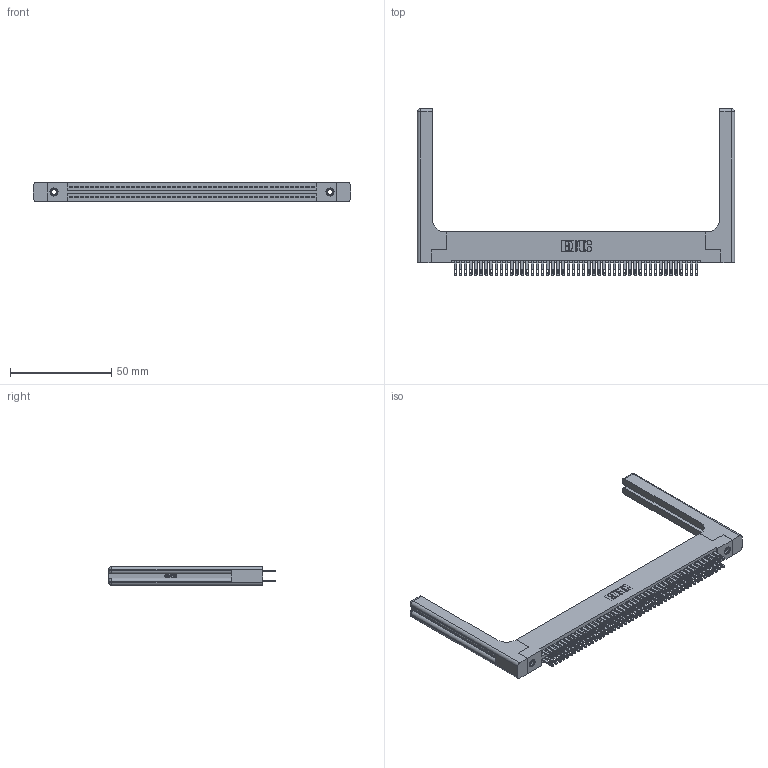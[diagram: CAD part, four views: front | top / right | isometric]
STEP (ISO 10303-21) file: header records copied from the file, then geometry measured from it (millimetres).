
FILE_DESCRIPTION (( 'STEP AP203' ), '1' );
FILE_NAME ('345-096-500-258.STEP', '2019-11-02T06:30:21', ( '' ), ( '' ), 'SwSTEP 2.0', 'SolidWorks 2016', '' );
FILE_SCHEMA (( 'CONFIG_CONTROL_DESIGN' ));
Length unit declared in the file: inch
Products named in the file (5): 345-096-500-258; 345 Part_Flush Mounting Lugs - 0.156 Dia-TH; 345-292-001_345-293-100; 345-220-058_345-220-058; 345-250-001_345-250-001-102
Assembly tree (101 placements, depth 2):
  345-096-500-258
    345 Part_Flush Mounting Lugs - 0.156 Dia-TH
    345-292-001_345-293-100  x96
    345-250-001_345-250-001-102  x2
    345-220-058_345-220-058  x2
Bounding box: 156.95 x 82.47 x 9.4 mm (x, y, z)
Volume: 24070.1 mm3; surface area: 29206.3 mm2
Topology: 101 solids, 101 shells, 4798 faces, 14543 edges, 9674 vertices
Faces by surface type: plane 2820, cylinder 1918, bspline 36, cone 12, sphere 8, torus 4
Entity records: 41966 total; most frequent: CARTESIAN_POINT 8021, ORIENTED_EDGE 6752, DIRECTION 6000, EDGE_CURVE 3376, VECTOR 2956, LINE 2956, VERTEX_POINT 2242, AXIS2_PLACEMENT_3D 1522
